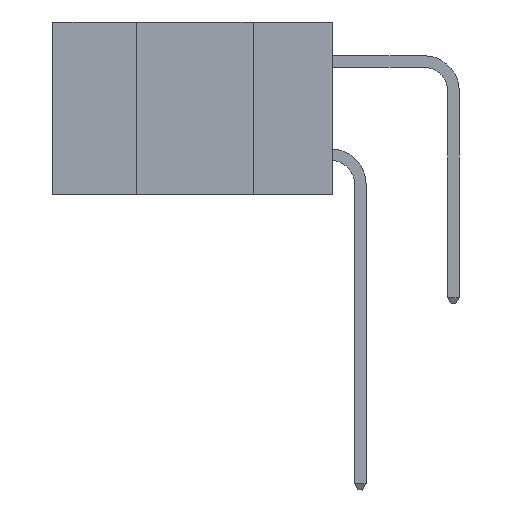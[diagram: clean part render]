
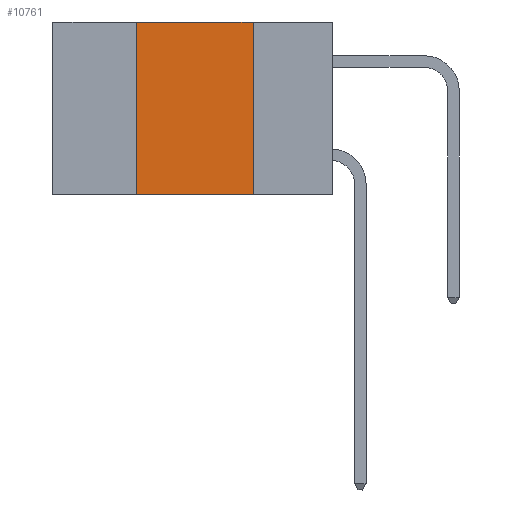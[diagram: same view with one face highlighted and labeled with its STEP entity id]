
A CAD part, left-side view. The second image highlights one B-rep face of the part: STEP entity #10761.
In plain terms, the highlighted planar face has unit normal (-1, 0, 0).
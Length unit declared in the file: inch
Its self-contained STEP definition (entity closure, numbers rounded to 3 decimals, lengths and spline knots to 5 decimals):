
#1380 = VERTEX_POINT ( 'NONE', #3854 ) ;
#1508 = FACE_OUTER_BOUND ( 'NONE', #4154, .T. ) ;
#1633 = DIRECTION ( 'NONE',  ( 0., -1., 0. ) ) ;
#1706 = EDGE_CURVE ( 'NONE', #9374, #13418, #10084, .T. ) ;
#1786 = DIRECTION ( 'NONE',  ( 1., 0., 0. ) ) ;
#2006 = EDGE_CURVE ( 'NONE', #15579, #1380, #8637, .T. ) ;
#2298 = VECTOR ( 'NONE', #7166, 39.37008 ) ;
#3115 = CARTESIAN_POINT ( 'NONE',  ( 0., 0.42, 0. ) ) ;
#3624 = DIRECTION ( 'NONE',  ( 0., 0., -1. ) ) ;
#3667 = CARTESIAN_POINT ( 'NONE',  ( 0., 0.17, 0. ) ) ;
#3854 = CARTESIAN_POINT ( 'NONE',  ( 0., 0.17, -0.37 ) ) ;
#4154 = EDGE_LOOP ( 'NONE', ( #15219, #4522, #16576, #11604 ) ) ;
#4522 = ORIENTED_EDGE ( 'NONE', *, *, #1706, .F. ) ;
#7166 = DIRECTION ( 'NONE',  ( 0., 0., 1. ) ) ;
#8637 = LINE ( 'NONE', #16007, #15145 ) ;
#9009 = EDGE_CURVE ( 'NONE', #13418, #1380, #13346, .T. ) ;
#9374 = VERTEX_POINT ( 'NONE', #14863 ) ;
#9831 = CARTESIAN_POINT ( 'NONE',  ( 0., 0.6, 0. ) ) ;
#9901 = VECTOR ( 'NONE', #3624, 39.37008 ) ;
#10084 = LINE ( 'NONE', #13821, #16884 ) ;
#10126 = AXIS2_PLACEMENT_3D ( 'NONE', #9831, #1786, #11160 ) ;
#10761 = ADVANCED_FACE ( 'NONE', ( #1508 ), #13676, .F. ) ;
#11160 = DIRECTION ( 'NONE',  ( 0., 0., -1. ) ) ;
#11604 = ORIENTED_EDGE ( 'NONE', *, *, #2006, .T. ) ;
#12854 = CARTESIAN_POINT ( 'NONE',  ( 0., 0.17, 0. ) ) ;
#13346 = LINE ( 'NONE', #12854, #9901 ) ;
#13418 = VERTEX_POINT ( 'NONE', #3667 ) ;
#13676 = PLANE ( 'NONE',  #10126 ) ;
#13821 = CARTESIAN_POINT ( 'NONE',  ( 0., 0.6, 0. ) ) ;
#14112 = DIRECTION ( 'NONE',  ( 0., -1., 0. ) ) ;
#14555 = CARTESIAN_POINT ( 'NONE',  ( 0., 0.42, -0.37 ) ) ;
#14863 = CARTESIAN_POINT ( 'NONE',  ( 0., 0.42, 0. ) ) ;
#15145 = VECTOR ( 'NONE', #1633, 39.37008 ) ;
#15219 = ORIENTED_EDGE ( 'NONE', *, *, #9009, .F. ) ;
#15579 = VERTEX_POINT ( 'NONE', #14555 ) ;
#16007 = CARTESIAN_POINT ( 'NONE',  ( 0., 0.6, -0.37 ) ) ;
#16306 = LINE ( 'NONE', #3115, #2298 ) ;
#16463 = EDGE_CURVE ( 'NONE', #15579, #9374, #16306, .T. ) ;
#16576 = ORIENTED_EDGE ( 'NONE', *, *, #16463, .F. ) ;
#16884 = VECTOR ( 'NONE', #14112, 39.37008 ) ;
